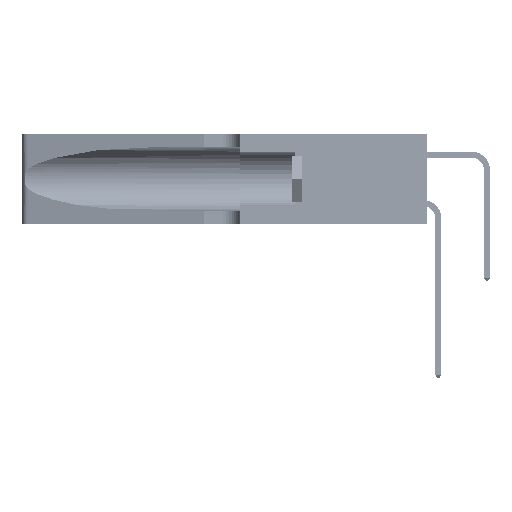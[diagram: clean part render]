
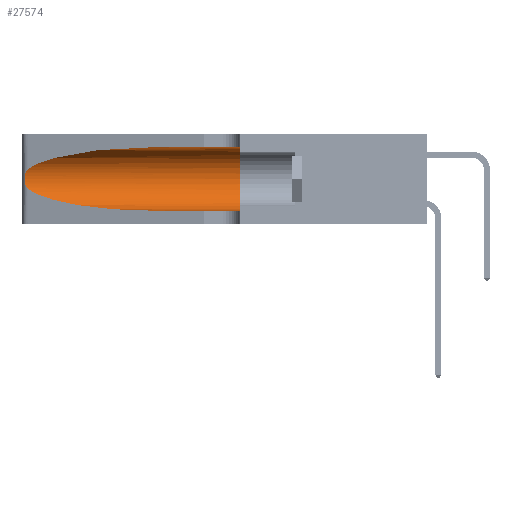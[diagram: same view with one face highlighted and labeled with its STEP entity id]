
A CAD part, left-side view. The second image highlights one B-rep face of the part: STEP entity #27574.
In plain terms, the highlighted cylindrical face has radius 3.308 mm (diameter 6.617 mm), a partial arc.
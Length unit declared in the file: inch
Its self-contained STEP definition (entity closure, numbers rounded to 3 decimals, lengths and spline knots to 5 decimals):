
#360 = CARTESIAN_POINT ( 'NONE',  ( 0.1305, 0.72297, 0.31525 ) ) ;
#399 = B_SPLINE_CURVE_WITH_KNOTS ( 'NONE', 3,
 ( #19125, #42149, #45981, #23022, #49805, #26901, #3642, #30754, #7582, #34607, #11517, #38456, #15380, #42314 ),
 .UNSPECIFIED., .F., .F.,
 ( 4, 2, 2, 2, 2, 2, 4 ),
 ( 0., 0.00027, 0.00053, 0.00107, 0.0016, 0.00187, 0.00214 ),
 .UNSPECIFIED. ) ;
#469 = CARTESIAN_POINT ( 'NONE',  ( 0.1305, 0.35, 0.185 ) ) ;
#2000 = CARTESIAN_POINT ( 'NONE',  ( 0.25487, 1.22718, 0.14631 ) ) ;
#2489 = EDGE_CURVE ( 'NONE', #7702, #38181, #12620, .T. ) ;
#3064 = EDGE_CURVE ( 'NONE', #33034, #17076, #399, .T. ) ;
#3642 = CARTESIAN_POINT ( 'NONE',  ( 0.26075, 1.23896, 0.19203 ) ) ;
#4372 = DIRECTION ( 'NONE',  ( 0., 0., 1. ) ) ;
#5313 = CARTESIAN_POINT ( 'NONE',  ( 0.1305, 0.72297, 0.05475 ) ) ;
#5866 = CARTESIAN_POINT ( 'NONE',  ( 0.1305, 0.35, 0.31525 ) ) ;
#7582 = CARTESIAN_POINT ( 'NONE',  ( 0.26017, 1.23833, 0.17102 ) ) ;
#7591 = FACE_OUTER_BOUND ( 'NONE', #40977, .T. ) ;
#7702 = VERTEX_POINT ( 'NONE', #5866 ) ;
#8402 = ORIENTED_EDGE ( 'NONE', *, *, #3064, .T. ) ;
#9208 = CARTESIAN_POINT ( 'NONE',  ( 0.25487, 1.22718, 0.22369 ) ) ;
#9214 = EDGE_CURVE ( 'NONE', #15757, #7702, #48000, .T. ) ;
#10700 = EDGE_CURVE ( 'NONE', #24145, #38181, #15465, .T. ) ;
#11517 = CARTESIAN_POINT ( 'NONE',  ( 0.25789, 1.23486, 0.15765 ) ) ;
#12384 = ORIENTED_EDGE ( 'NONE', *, *, #10700, .T. ) ;
#12620 = CIRCLE ( 'NONE', #20824, 0.13025 ) ;
#12626 = CARTESIAN_POINT ( 'NONE',  ( 0.2373, 1.15595, 0.28018 ) ) ;
#13752 = ORIENTED_EDGE ( 'NONE', *, *, #2489, .F. ) ;
#14368 = DIRECTION ( 'NONE',  ( 0., 0., -1. ) ) ;
#15380 = CARTESIAN_POINT ( 'NONE',  ( 0.25555, 1.22993, 0.14849 ) ) ;
#15465 = LINE ( 'NONE', #21275, #43729 ) ;
#15757 = VERTEX_POINT ( 'NONE', #360 ) ;
#16861 = CARTESIAN_POINT ( 'NONE',  ( 0.25487, 1.22718, 0.14631 ) ) ;
#17076 = VERTEX_POINT ( 'NONE', #2000 ) ;
#17336 = VECTOR ( 'NONE', #49166, 39.37008 ) ;
#19125 = CARTESIAN_POINT ( 'NONE',  ( 0.25487, 1.22718, 0.22369 ) ) ;
#19887 = ORIENTED_EDGE ( 'NONE', *, *, #9214, .F. ) ;
#20824 = AXIS2_PLACEMENT_3D ( 'NONE', #469, #27614, #4372 ) ;
#21275 = CARTESIAN_POINT ( 'NONE',  ( 0.1305, 1.61858, 0.05475 ) ) ;
#22184 = DIRECTION ( 'NONE',  ( 0., -1., 0. ) ) ;
#23022 = CARTESIAN_POINT ( 'NONE',  ( 0.25787, 1.23484, 0.2124 ) ) ;
#24145 = VERTEX_POINT ( 'NONE', #24792 ) ;
#24792 = CARTESIAN_POINT ( 'NONE',  ( 0.1305, 0.72297, 0.05475 ) ) ;
#25130 = DIRECTION ( 'NONE',  ( 0., -1., 0. ) ) ;
#25308 =( BOUNDED_CURVE ( )  B_SPLINE_CURVE ( 3, ( #16861, #47609, #28541, #5313 ),
 .UNSPECIFIED., .F., .T. ) 
 B_SPLINE_CURVE_WITH_KNOTS ( ( 4, 4 ),
 ( 3.44316, 4.71239 ),
 .UNSPECIFIED. ) 
 CURVE ( )  GEOMETRIC_REPRESENTATION_ITEM ( )  RATIONAL_B_SPLINE_CURVE ( ( 1., 0.87, 0.87, 1. ) ) 
 REPRESENTATION_ITEM ( '' )  );
#26866 = AXIS2_PLACEMENT_3D ( 'NONE', #45149, #22184, #14368 ) ;
#26901 = CARTESIAN_POINT ( 'NONE',  ( 0.26018, 1.23835, 0.19895 ) ) ;
#26986 = CYLINDRICAL_SURFACE ( 'NONE', #26866, 0.13025 ) ;
#27574 = ADVANCED_FACE ( 'NONE', ( #7591 ), #26986, .F. ) ;
#27614 = DIRECTION ( 'NONE',  ( 0., 1., 0. ) ) ;
#28541 = CARTESIAN_POINT ( 'NONE',  ( 0.18966, 0.96281, 0.05475 ) ) ;
#30754 = CARTESIAN_POINT ( 'NONE',  ( 0.26075, 1.23896, 0.178 ) ) ;
#31849 = CARTESIAN_POINT ( 'NONE',  ( 0.1305, 0.72297, 0.31525 ) ) ;
#33034 = VERTEX_POINT ( 'NONE', #9208 ) ;
#34607 = CARTESIAN_POINT ( 'NONE',  ( 0.25856, 1.23593, 0.16098 ) ) ;
#35718 = CARTESIAN_POINT ( 'NONE',  ( 0.18966, 0.96281, 0.31525 ) ) ;
#38181 = VERTEX_POINT ( 'NONE', #43762 ) ;
#38456 = CARTESIAN_POINT ( 'NONE',  ( 0.25639, 1.23186, 0.15144 ) ) ;
#39544 = CARTESIAN_POINT ( 'NONE',  ( 0.25487, 1.22718, 0.22369 ) ) ;
#40977 = EDGE_LOOP ( 'NONE', ( #47718, #8402, #43308, #12384, #13752, #19887 ) ) ;
#42149 = CARTESIAN_POINT ( 'NONE',  ( 0.25555, 1.22994, 0.2215 ) ) ;
#42314 = CARTESIAN_POINT ( 'NONE',  ( 0.25487, 1.22718, 0.14631 ) ) ;
#43308 = ORIENTED_EDGE ( 'NONE', *, *, #44001, .T. ) ;
#43729 = VECTOR ( 'NONE', #25130, 39.37008 ) ;
#43762 = CARTESIAN_POINT ( 'NONE',  ( 0.1305, 0.35, 0.05475 ) ) ;
#44001 = EDGE_CURVE ( 'NONE', #17076, #24145, #25308, .T. ) ;
#45149 = CARTESIAN_POINT ( 'NONE',  ( 0.1305, 1.61858, 0.185 ) ) ;
#45340 = CARTESIAN_POINT ( 'NONE',  ( 0.1305, 1.61858, 0.31525 ) ) ;
#45981 = CARTESIAN_POINT ( 'NONE',  ( 0.25639, 1.23184, 0.21858 ) ) ;
#47609 = CARTESIAN_POINT ( 'NONE',  ( 0.2373, 1.15595, 0.08982 ) ) ;
#47690 = EDGE_CURVE ( 'NONE', #15757, #33034, #48312, .T. ) ;
#47718 = ORIENTED_EDGE ( 'NONE', *, *, #47690, .T. ) ;
#48000 = LINE ( 'NONE', #45340, #17336 ) ;
#48312 =( BOUNDED_CURVE ( )  B_SPLINE_CURVE ( 3, ( #31849, #35718, #12626, #39544 ),
 .UNSPECIFIED., .F., .T. ) 
 B_SPLINE_CURVE_WITH_KNOTS ( ( 4, 4 ),
 ( 1.5708, 2.84003 ),
 .UNSPECIFIED. ) 
 CURVE ( )  GEOMETRIC_REPRESENTATION_ITEM ( )  RATIONAL_B_SPLINE_CURVE ( ( 1., 0.87, 0.87, 1. ) ) 
 REPRESENTATION_ITEM ( '' )  );
#49166 = DIRECTION ( 'NONE',  ( 0., -1., 0. ) ) ;
#49805 = CARTESIAN_POINT ( 'NONE',  ( 0.25854, 1.2359, 0.20912 ) ) ;
